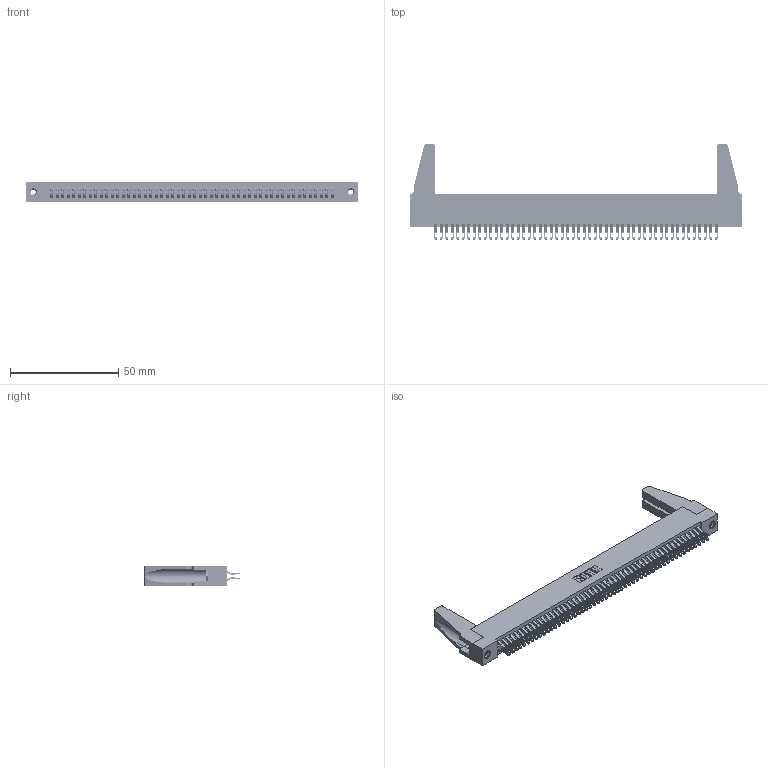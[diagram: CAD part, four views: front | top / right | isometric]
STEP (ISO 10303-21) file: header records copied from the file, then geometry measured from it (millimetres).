
FILE_DESCRIPTION (( 'STEP AP203' ), '1' );
FILE_NAME ('345-104-555-288.STEP', '2019-11-03T12:34:57', ( '' ), ( '' ), 'SwSTEP 2.0', 'SolidWorks 2016', '' );
FILE_SCHEMA (( 'CONFIG_CONTROL_DESIGN' ));
Length unit declared in the file: inch
Products named in the file (5): 345-104-555-288; 345-292-001_555 Tail; 345 Part_Flush Mounting Lugs - 0.156 Dia-TH; 345-220-078_345-220-088; 345-250-001_345-250-001-102
Assembly tree (109 placements, depth 2):
  345-104-555-288
    345 Part_Flush Mounting Lugs - 0.156 Dia-TH
    345-292-001_555 Tail  x104
    345-250-001_345-250-001-102  x2
    345-220-078_345-220-088  x2
Bounding box: 153.31 x 43.99 x 9.4 mm (x, y, z)
Volume: 18540 mm3; surface area: 26962.6 mm2
Topology: 109 solids, 109 shells, 6074 faces, 19063 edges, 12698 vertices
Faces by surface type: plane 3376, cylinder 2682, cone 12, torus 4
Entity records: 41928 total; most frequent: CARTESIAN_POINT 7048, ORIENTED_EDGE 6912, DIRECTION 6176, EDGE_CURVE 3456, LINE 3054, VECTOR 3054, VERTEX_POINT 2298, AXIS2_PLACEMENT_3D 1561
